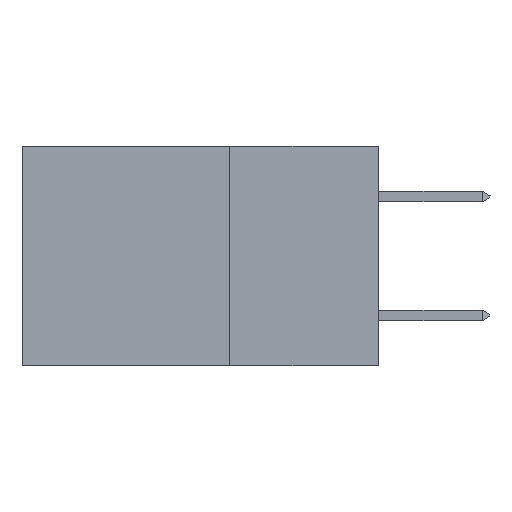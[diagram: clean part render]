
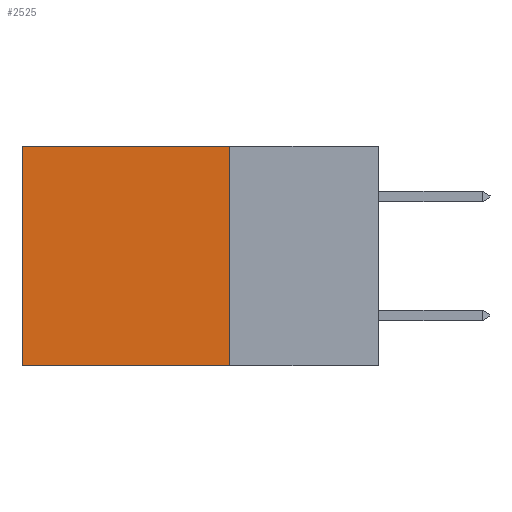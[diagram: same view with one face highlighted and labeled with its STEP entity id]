
A CAD part, left-side view. The second image highlights one B-rep face of the part: STEP entity #2525.
In plain terms, the highlighted planar face has unit normal (-1, 0, 0).
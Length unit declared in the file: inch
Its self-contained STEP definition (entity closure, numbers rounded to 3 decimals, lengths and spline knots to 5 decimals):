
#337 = DIRECTION ( 'NONE',  ( 0., 1., 0. ) ) ;
#428 = CARTESIAN_POINT ( 'NONE',  ( 0.2615, 0.25, 0. ) ) ;
#992 = CARTESIAN_POINT ( 'NONE',  ( 0.2615, 0.25, -0.37 ) ) ;
#1159 = CARTESIAN_POINT ( 'NONE',  ( 0.2615, 0.25, -0.37 ) ) ;
#1285 = EDGE_CURVE ( 'NONE', #3956, #1779, #6387, .T. ) ;
#1398 = CARTESIAN_POINT ( 'NONE',  ( 0.2615, 0.6, -0.37 ) ) ;
#1425 = ORIENTED_EDGE ( 'NONE', *, *, #8529, .F. ) ;
#1779 = VERTEX_POINT ( 'NONE', #9990 ) ;
#2009 = VERTEX_POINT ( 'NONE', #2735 ) ;
#2525 = ADVANCED_FACE ( 'NONE', ( #6654 ), #7295, .F. ) ;
#2735 = CARTESIAN_POINT ( 'NONE',  ( 0.2615, 0.6, -0.37 ) ) ;
#3956 = VERTEX_POINT ( 'NONE', #428 ) ;
#4039 = VECTOR ( 'NONE', #5556, 39.37008 ) ;
#4669 = DIRECTION ( 'NONE',  ( 0., 0., -1. ) ) ;
#4891 = DIRECTION ( 'NONE',  ( 0., 0., -1. ) ) ;
#5309 = VECTOR ( 'NONE', #337, 39.37008 ) ;
#5556 = DIRECTION ( 'NONE',  ( 0., 1., 0. ) ) ;
#5761 = AXIS2_PLACEMENT_3D ( 'NONE', #7416, #8245, #5772 ) ;
#5772 = DIRECTION ( 'NONE',  ( 0., 0., -1. ) ) ;
#6294 = VECTOR ( 'NONE', #4891, 39.37008 ) ;
#6387 = LINE ( 'NONE', #10137, #4039 ) ;
#6654 = FACE_OUTER_BOUND ( 'NONE', #10948, .T. ) ;
#6723 = CARTESIAN_POINT ( 'NONE',  ( 0.2615, 0.25, -0.37 ) ) ;
#7079 = ORIENTED_EDGE ( 'NONE', *, *, #9919, .T. ) ;
#7295 = PLANE ( 'NONE',  #5761 ) ;
#7394 = LINE ( 'NONE', #1159, #9876 ) ;
#7416 = CARTESIAN_POINT ( 'NONE',  ( 0.2615, 0.25, -0.37 ) ) ;
#7484 = ORIENTED_EDGE ( 'NONE', *, *, #1285, .T. ) ;
#8087 = VERTEX_POINT ( 'NONE', #992 ) ;
#8245 = DIRECTION ( 'NONE',  ( 1., 0., 0. ) ) ;
#8277 = EDGE_CURVE ( 'NONE', #8087, #2009, #8483, .T. ) ;
#8483 = LINE ( 'NONE', #6723, #5309 ) ;
#8529 = EDGE_CURVE ( 'NONE', #3956, #8087, #7394, .T. ) ;
#9359 = LINE ( 'NONE', #1398, #6294 ) ;
#9876 = VECTOR ( 'NONE', #4669, 39.37008 ) ;
#9919 = EDGE_CURVE ( 'NONE', #1779, #2009, #9359, .T. ) ;
#9990 = CARTESIAN_POINT ( 'NONE',  ( 0.2615, 0.6, 0. ) ) ;
#10137 = CARTESIAN_POINT ( 'NONE',  ( 0.2615, 0.25, 0. ) ) ;
#10561 = ORIENTED_EDGE ( 'NONE', *, *, #8277, .F. ) ;
#10948 = EDGE_LOOP ( 'NONE', ( #7079, #10561, #1425, #7484 ) ) ;
